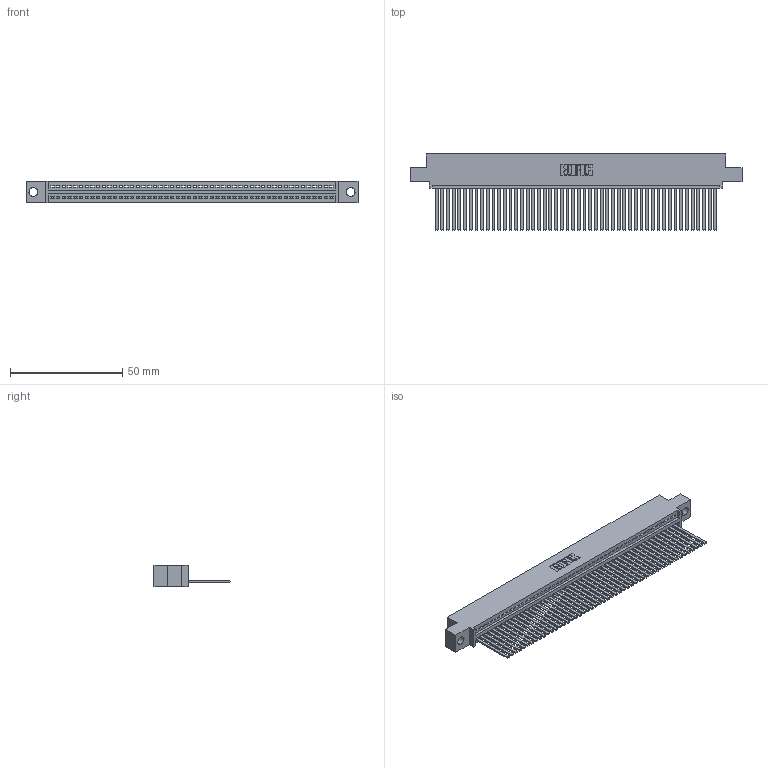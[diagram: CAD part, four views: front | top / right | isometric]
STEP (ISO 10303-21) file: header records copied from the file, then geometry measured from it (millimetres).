
FILE_DESCRIPTION (( 'STEP AP203' ), '1' );
FILE_NAME ('345-050-544-404.STEP', '2021-05-26T15:21:55', ( '' ), ( '' ), 'SwSTEP 2.0', 'SolidWorks 2020', '' );
FILE_SCHEMA (( 'CONFIG_CONTROL_DESIGN' ));
Length unit declared in the file: inch
Products named in the file (3): 345-050-544-404; 345-292-001_345-293-144; 345 Part_0.110 Offset - 0.156 Dia-TI
Assembly tree (51 placements, depth 2):
  345-050-544-404
    345 Part_0.110 Offset - 0.156 Dia-TI
    345-292-001_345-293-144  x50
Bounding box: 148.21 x 33.96 x 9.4 mm (x, y, z)
Volume: 14542.3 mm3; surface area: 21096.9 mm2
Topology: 51 solids, 51 shells, 2744 faces, 8289 edges, 5458 vertices
Faces by surface type: plane 1898, cylinder 846
Entity records: 36921 total; most frequent: CARTESIAN_POINT 6404, ORIENTED_EDGE 6386, DIRECTION 5577, EDGE_CURVE 3193, LINE 2865, VECTOR 2865, VERTEX_POINT 2126, AXIS2_PLACEMENT_3D 1356
